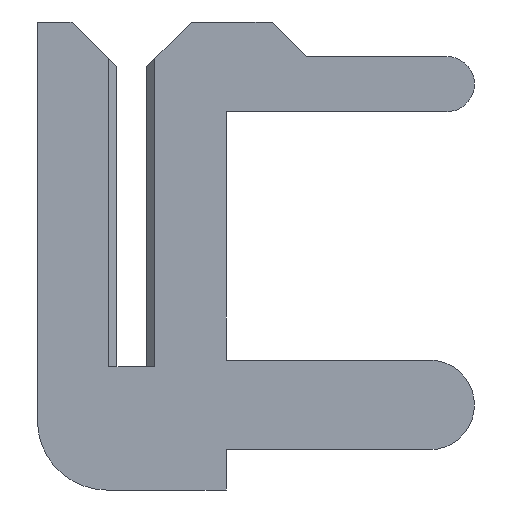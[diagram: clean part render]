
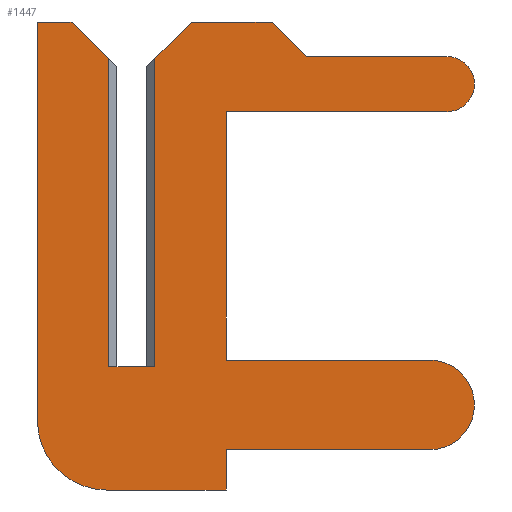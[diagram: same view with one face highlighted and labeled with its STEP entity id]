
A CAD part, left-side view. The second image highlights one B-rep face of the part: STEP entity #1447.
In plain terms, the highlighted planar face has unit normal (-1, 0, 0).
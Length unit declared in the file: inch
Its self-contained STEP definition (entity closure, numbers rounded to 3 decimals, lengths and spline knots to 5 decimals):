
#28 = ORIENTED_EDGE ( 'NONE', *, *, #391, .F. ) ;
#29 = EDGE_CURVE ( 'NONE', #1311, #1119, #1274, .T. ) ;
#38 = CIRCLE ( 'NONE', #602, 0.012 ) ;
#42 = VECTOR ( 'NONE', #259, 39.37008 ) ;
#77 = DIRECTION ( 'NONE',  ( 0., -1., 0. ) ) ;
#83 = CARTESIAN_POINT ( 'NONE',  ( -0.01, -0.061, 0.15 ) ) ;
#108 = DIRECTION ( 'NONE',  ( 0., -1., 0. ) ) ;
#117 = VECTOR ( 'NONE', #124, 39.37008 ) ;
#119 = CARTESIAN_POINT ( 'NONE',  ( -0.01, -0.137, 0.111 ) ) ;
#122 = DIRECTION ( 'NONE',  ( 1., 0., 0. ) ) ;
#124 = DIRECTION ( 'NONE',  ( 0., -0.707, 0.707 ) ) ;
#139 = DIRECTION ( 'NONE',  ( 0., -1., 0. ) ) ;
#145 = CARTESIAN_POINT ( 'NONE',  ( -0.01, 0.0065, 0.1305 ) ) ;
#152 = VERTEX_POINT ( 'NONE', #1385 ) ;
#172 = LINE ( 'NONE', #503, #1244 ) ;
#176 = DIRECTION ( 'NONE',  ( 1., 0., 0. ) ) ;
#182 = DIRECTION ( 'NONE',  ( 0., -1., 0. ) ) ;
#201 = DIRECTION ( 'NONE',  ( 0., 0., 1. ) ) ;
#208 = CARTESIAN_POINT ( 'NONE',  ( -0.01, -0.01, 0.134 ) ) ;
#210 = ORIENTED_EDGE ( 'NONE', *, *, #1111, .F. ) ;
#228 = EDGE_LOOP ( 'NONE', ( #896, #1354, #1437, #1455, #1416, #242, #1230, #1032, #816, #1102, #819, #210, #1004, #1149, #28, #974, #869, #1388, #570 ) ) ;
#242 = ORIENTED_EDGE ( 'NONE', *, *, #1427, .F. ) ;
#249 = EDGE_CURVE ( 'NONE', #1119, #1092, #1037, .T. ) ;
#258 = VECTOR ( 'NONE', #108, 39.37008 ) ;
#259 = DIRECTION ( 'NONE',  ( 0., -0.707, -0.707 ) ) ;
#263 = VERTEX_POINT ( 'NONE', #319 ) ;
#273 = VERTEX_POINT ( 'NONE', #1151 ) ;
#281 = VECTOR ( 'NONE', #139, 39.37008 ) ;
#283 = VECTOR ( 'NONE', #1167, 39.37008 ) ;
#284 = EDGE_CURVE ( 'NONE', #568, #937, #38, .T. ) ;
#286 = VERTEX_POINT ( 'NONE', #905 ) ;
#303 = LINE ( 'NONE', #1283, #258 ) ;
#308 = EDGE_CURVE ( 'NONE', #152, #568, #1122, .T. ) ;
#313 = DIRECTION ( 'NONE',  ( 0., 0., -1. ) ) ;
#319 = CARTESIAN_POINT ( 'NONE',  ( -0.01, -0.041, 0.111 ) ) ;
#323 = VERTEX_POINT ( 'NONE', #83 ) ;
#327 = CIRCLE ( 'NONE', #1012, 0.03 ) ;
#331 = PLANE ( 'NONE',  #1449 ) ;
#350 = CARTESIAN_POINT ( 'NONE',  ( -0.01, -0.137, 0.123 ) ) ;
#352 = CARTESIAN_POINT ( 'NONE',  ( -0.01, 0.01, 0. ) ) ;
#380 = VECTOR ( 'NONE', #313, 39.37008 ) ;
#391 = EDGE_CURVE ( 'NONE', #937, #263, #591, .T. ) ;
#394 = CARTESIAN_POINT ( 'NONE',  ( -0.01, -0.1295, -0.0165 ) ) ;
#395 = CARTESIAN_POINT ( 'NONE',  ( -0.01, -0.137, 0.135 ) ) ;
#399 = VECTOR ( 'NONE', #182, 39.37008 ) ;
#406 = EDGE_CURVE ( 'NONE', #1330, #1482, #877, .T. ) ;
#415 = EDGE_CURVE ( 'NONE', #709, #323, #303, .T. ) ;
#423 = VERTEX_POINT ( 'NONE', #352 ) ;
#442 = DIRECTION ( 'NONE',  ( 0., 0., 1. ) ) ;
#458 = DIRECTION ( 'NONE',  ( 0., -1., 0. ) ) ;
#462 = VERTEX_POINT ( 'NONE', #728 ) ;
#470 = LINE ( 'NONE', #1499, #745 ) ;
#493 = EDGE_CURVE ( 'NONE', #462, #676, #1028, .T. ) ;
#503 = CARTESIAN_POINT ( 'NONE',  ( -0.01, 0.041, 0.15 ) ) ;
#508 = VECTOR ( 'NONE', #458, 39.37008 ) ;
#511 = DIRECTION ( 'NONE',  ( 0., 0., 1. ) ) ;
#519 = CARTESIAN_POINT ( 'NONE',  ( -0.01, 0.01, 0.134 ) ) ;
#521 = EDGE_CURVE ( 'NONE', #323, #152, #971, .T. ) ;
#522 = VECTOR ( 'NONE', #1475, 39.37008 ) ;
#530 = LINE ( 'NONE', #1436, #117 ) ;
#533 = DIRECTION ( 'NONE',  ( 0., 0., -1. ) ) ;
#552 = DIRECTION ( 'NONE',  ( -1., 0., 0. ) ) ;
#562 = DIRECTION ( 'NONE',  ( 0., 0., 1. ) ) ;
#568 = VERTEX_POINT ( 'NONE', #395 ) ;
#570 = ORIENTED_EDGE ( 'NONE', *, *, #415, .F. ) ;
#582 = EDGE_CURVE ( 'NONE', #1185, #1192, #172, .T. ) ;
#591 = LINE ( 'NONE', #1038, #283 ) ;
#602 = AXIS2_PLACEMENT_3D ( 'NONE', #350, #680, #562 ) ;
#606 = LINE ( 'NONE', #1200, #522 ) ;
#637 = EDGE_CURVE ( 'NONE', #1330, #709, #530, .T. ) ;
#649 = DIRECTION ( 'NONE',  ( 0., 0., 1. ) ) ;
#663 = CARTESIAN_POINT ( 'NONE',  ( -0.01, -0.041, -0.036 ) ) ;
#670 = DIRECTION ( 'NONE',  ( 0., 1., 0. ) ) ;
#676 = VERTEX_POINT ( 'NONE', #519 ) ;
#680 = DIRECTION ( 'NONE',  ( 1., 0., 0. ) ) ;
#709 = VERTEX_POINT ( 'NONE', #743 ) ;
#727 = LINE ( 'NONE', #1383, #929 ) ;
#728 = CARTESIAN_POINT ( 'NONE',  ( -0.01, 0.026, 0.15 ) ) ;
#743 = CARTESIAN_POINT ( 'NONE',  ( -0.01, -0.026, 0.15 ) ) ;
#745 = VECTOR ( 'NONE', #201, 39.37008 ) ;
#812 = CARTESIAN_POINT ( 'NONE',  ( -0.01, 0.0065, 0. ) ) ;
#816 = ORIENTED_EDGE ( 'NONE', *, *, #1146, .F. ) ;
#818 = VECTOR ( 'NONE', #670, 39.37008 ) ;
#819 = ORIENTED_EDGE ( 'NONE', *, *, #29, .F. ) ;
#829 = CARTESIAN_POINT ( 'NONE',  ( -0.01, 0.011, -0.0235 ) ) ;
#845 = VECTOR ( 'NONE', #1428, 39.37008 ) ;
#867 = CARTESIAN_POINT ( 'NONE',  ( -0.01, -0.041, 0.003 ) ) ;
#869 = ORIENTED_EDGE ( 'NONE', *, *, #308, .F. ) ;
#875 = CARTESIAN_POINT ( 'NONE',  ( -0.01, 0.041, 0.15 ) ) ;
#877 = LINE ( 'NONE', #920, #1479 ) ;
#892 = CARTESIAN_POINT ( 'NONE',  ( -0.01, -0.137, 0.135 ) ) ;
#896 = ORIENTED_EDGE ( 'NONE', *, *, #637, .F. ) ;
#905 = CARTESIAN_POINT ( 'NONE',  ( -0.01, -0.1295, 0.003 ) ) ;
#910 = LINE ( 'NONE', #1484, #399 ) ;
#920 = CARTESIAN_POINT ( 'NONE',  ( -0.01, -0.01, 0.15 ) ) ;
#929 = VECTOR ( 'NONE', #77, 39.37008 ) ;
#935 = DIRECTION ( 'NONE',  ( 0., 0., -1. ) ) ;
#937 = VERTEX_POINT ( 'NONE', #119 ) ;
#938 = DIRECTION ( 'NONE',  ( 0., 0., 1. ) ) ;
#945 = EDGE_CURVE ( 'NONE', #423, #1482, #1272, .T. ) ;
#961 = CARTESIAN_POINT ( 'NONE',  ( -0.01, -0.076, 0.135 ) ) ;
#965 = CARTESIAN_POINT ( 'NONE',  ( -0.01, -0.041, -0.036 ) ) ;
#971 = LINE ( 'NONE', #961, #42 ) ;
#974 = ORIENTED_EDGE ( 'NONE', *, *, #284, .F. ) ;
#977 = CARTESIAN_POINT ( 'NONE',  ( -0.01, -0.041, -0.0535 ) ) ;
#985 = AXIS2_PLACEMENT_3D ( 'NONE', #394, #176, #649 ) ;
#987 = CARTESIAN_POINT ( 'NONE',  ( -0.01, -0.041, -0.0535 ) ) ;
#993 = EDGE_CURVE ( 'NONE', #273, #1185, #327, .T. ) ;
#1000 = CARTESIAN_POINT ( 'NONE',  ( -0.01, -0.041, 0.003 ) ) ;
#1001 = LINE ( 'NONE', #1000, #1289 ) ;
#1004 = ORIENTED_EDGE ( 'NONE', *, *, #1222, .F. ) ;
#1007 = CARTESIAN_POINT ( 'NONE',  ( -0.01, 0.011, -0.0235 ) ) ;
#1012 = AXIS2_PLACEMENT_3D ( 'NONE', #829, #122, #938 ) ;
#1028 = LINE ( 'NONE', #145, #845 ) ;
#1032 = ORIENTED_EDGE ( 'NONE', *, *, #993, .F. ) ;
#1037 = LINE ( 'NONE', #987, #380 ) ;
#1038 = CARTESIAN_POINT ( 'NONE',  ( -0.01, -0.041, 0.111 ) ) ;
#1092 = VERTEX_POINT ( 'NONE', #977 ) ;
#1102 = ORIENTED_EDGE ( 'NONE', *, *, #249, .F. ) ;
#1106 = CARTESIAN_POINT ( 'NONE',  ( -0.01, 0.041, -0.0235 ) ) ;
#1111 = EDGE_CURVE ( 'NONE', #286, #1311, #1451, .T. ) ;
#1119 = VERTEX_POINT ( 'NONE', #965 ) ;
#1122 = LINE ( 'NONE', #892, #508 ) ;
#1146 = EDGE_CURVE ( 'NONE', #1092, #273, #606, .T. ) ;
#1149 = ORIENTED_EDGE ( 'NONE', *, *, #1163, .F. ) ;
#1151 = CARTESIAN_POINT ( 'NONE',  ( -0.01, 0.011, -0.0535 ) ) ;
#1163 = EDGE_CURVE ( 'NONE', #263, #1213, #1001, .T. ) ;
#1167 = DIRECTION ( 'NONE',  ( 0., 1., 0. ) ) ;
#1185 = VERTEX_POINT ( 'NONE', #1106 ) ;
#1192 = VERTEX_POINT ( 'NONE', #875 ) ;
#1200 = CARTESIAN_POINT ( 'NONE',  ( -0.01, 0.011, -0.0535 ) ) ;
#1213 = VERTEX_POINT ( 'NONE', #867 ) ;
#1222 = EDGE_CURVE ( 'NONE', #1213, #286, #910, .T. ) ;
#1230 = ORIENTED_EDGE ( 'NONE', *, *, #582, .F. ) ;
#1244 = VECTOR ( 'NONE', #511, 39.37008 ) ;
#1272 = LINE ( 'NONE', #812, #281 ) ;
#1274 = LINE ( 'NONE', #663, #818 ) ;
#1275 = CARTESIAN_POINT ( 'NONE',  ( -0.01, -0.1295, -0.036 ) ) ;
#1283 = CARTESIAN_POINT ( 'NONE',  ( -0.01, -0.026, 0.15 ) ) ;
#1285 = CARTESIAN_POINT ( 'NONE',  ( -0.01, -0.01, 0. ) ) ;
#1289 = VECTOR ( 'NONE', #533, 39.37008 ) ;
#1311 = VERTEX_POINT ( 'NONE', #1275 ) ;
#1330 = VERTEX_POINT ( 'NONE', #208 ) ;
#1354 = ORIENTED_EDGE ( 'NONE', *, *, #406, .T. ) ;
#1383 = CARTESIAN_POINT ( 'NONE',  ( -0.01, 0.026, 0.15 ) ) ;
#1385 = CARTESIAN_POINT ( 'NONE',  ( -0.01, -0.076, 0.135 ) ) ;
#1388 = ORIENTED_EDGE ( 'NONE', *, *, #521, .F. ) ;
#1392 = FACE_OUTER_BOUND ( 'NONE', #228, .T. ) ;
#1416 = ORIENTED_EDGE ( 'NONE', *, *, #493, .F. ) ;
#1427 = EDGE_CURVE ( 'NONE', #1192, #462, #727, .T. ) ;
#1428 = DIRECTION ( 'NONE',  ( 0., -0.707, -0.707 ) ) ;
#1436 = CARTESIAN_POINT ( 'NONE',  ( -0.01, -0.0065, 0.1305 ) ) ;
#1437 = ORIENTED_EDGE ( 'NONE', *, *, #945, .F. ) ;
#1441 = EDGE_CURVE ( 'NONE', #423, #676, #470, .T. ) ;
#1447 = ADVANCED_FACE ( 'NONE', ( #1392 ), #331, .T. ) ;
#1449 = AXIS2_PLACEMENT_3D ( 'NONE', #1007, #552, #442 ) ;
#1451 = CIRCLE ( 'NONE', #985, 0.0195 ) ;
#1455 = ORIENTED_EDGE ( 'NONE', *, *, #1441, .T. ) ;
#1475 = DIRECTION ( 'NONE',  ( 0., 1., 0. ) ) ;
#1479 = VECTOR ( 'NONE', #935, 39.37008 ) ;
#1482 = VERTEX_POINT ( 'NONE', #1285 ) ;
#1484 = CARTESIAN_POINT ( 'NONE',  ( -0.01, -0.1295, 0.003 ) ) ;
#1499 = CARTESIAN_POINT ( 'NONE',  ( -0.01, 0.01, -0.0235 ) ) ;
